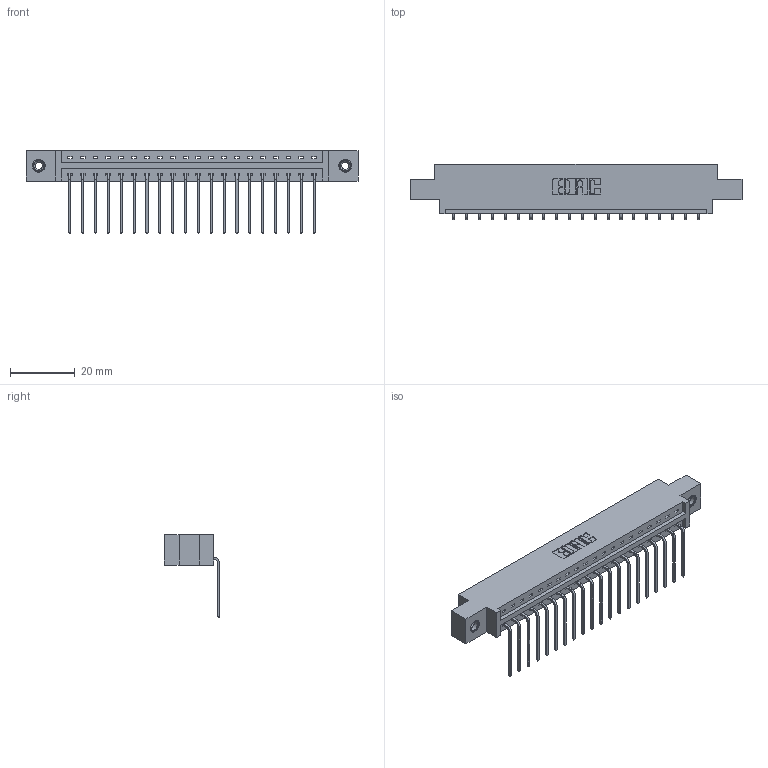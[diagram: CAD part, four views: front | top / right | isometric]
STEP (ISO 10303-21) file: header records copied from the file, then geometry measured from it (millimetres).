
FILE_DESCRIPTION (( 'STEP AP203' ), '1' );
FILE_NAME ('337-020-559-608.STEP', '2018-08-05T10:39:49', ( '' ), ( '' ), 'SwSTEP 2.0', 'SolidWorks 2016', '' );
FILE_SCHEMA (( 'CONFIG_CONTROL_DESIGN' ));
Length unit declared in the file: inch
Products named in the file (4): 337 Part_0.170 Offset - 0.156 Dia-TI; 345-292-001_558 559 Tail - 1; 345-250-001_345-250-003-102; 337-020-559-608
Assembly tree (23 placements, depth 2):
  337-020-559-608
    337 Part_0.170 Offset - 0.156 Dia-TI
    345-292-001_558 559 Tail - 1  x20
    345-250-001_345-250-003-102  x2
Bounding box: 102.26 x 17.09 x 25.53 mm (x, y, z)
Volume: 10295.6 mm3; surface area: 11052.3 mm2
Topology: 23 solids, 23 shells, 1458 faces, 4339 edges, 2858 vertices
Faces by surface type: plane 1066, cylinder 376, cone 12, torus 4
Entity records: 19114 total; most frequent: CARTESIAN_POINT 3309, ORIENTED_EDGE 3258, DIRECTION 2863, EDGE_CURVE 1629, LINE 1481, VECTOR 1481, VERTEX_POINT 1080, AXIS2_PLACEMENT_3D 691
